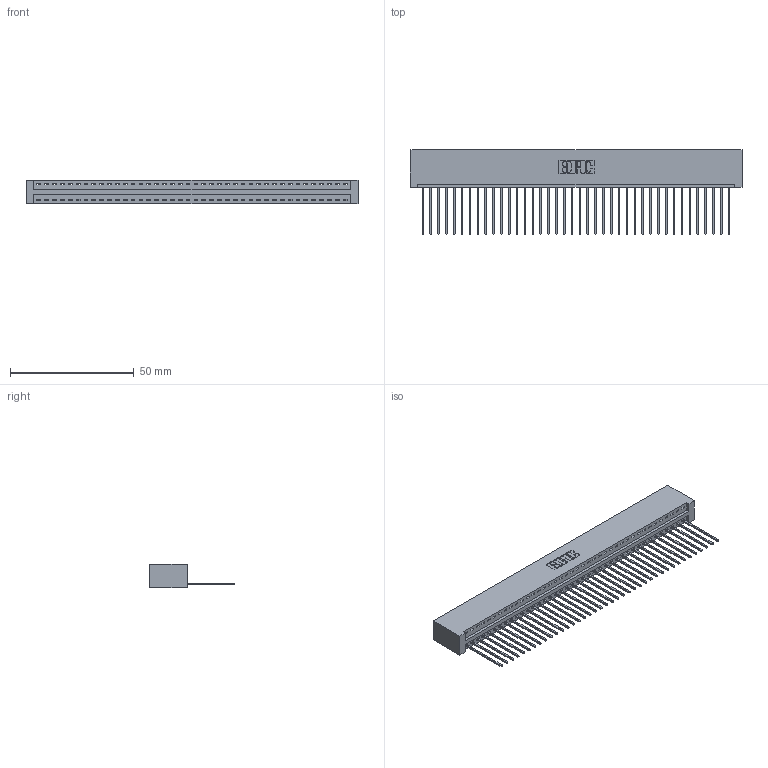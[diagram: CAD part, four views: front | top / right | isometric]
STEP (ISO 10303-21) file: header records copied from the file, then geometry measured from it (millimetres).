
FILE_DESCRIPTION (( 'STEP AP203' ), '1' );
FILE_NAME ('346-040-541-101.STEP', '2022-05-07T09:55:29', ( '' ), ( '' ), 'SwSTEP 2.0', 'SolidWorks 2020', '' );
FILE_SCHEMA (( 'CONFIG_CONTROL_DESIGN' ));
Length unit declared in the file: inch
Products named in the file (3): 345-292-001_345-293-141; 346 Part_No Mounting Lugs; 346-040-541-101
Assembly tree (41 placements, depth 2):
  346-040-541-101
    346 Part_No Mounting Lugs
    345-292-001_345-293-141  x40
Bounding box: 134.24 x 34.29 x 9.4 mm (x, y, z)
Volume: 13517.3 mm3; surface area: 17736.9 mm2
Topology: 41 solids, 41 shells, 2434 faces, 7345 edges, 4842 vertices
Faces by surface type: plane 1672, cylinder 762
Entity records: 24835 total; most frequent: CARTESIAN_POINT 4264, ORIENTED_EDGE 4238, DIRECTION 3759, EDGE_CURVE 2119, VECTOR 1835, LINE 1835, VERTEX_POINT 1410, AXIS2_PLACEMENT_3D 962
